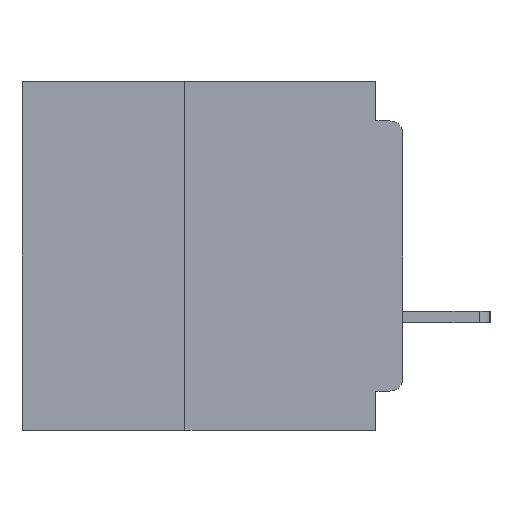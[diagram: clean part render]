
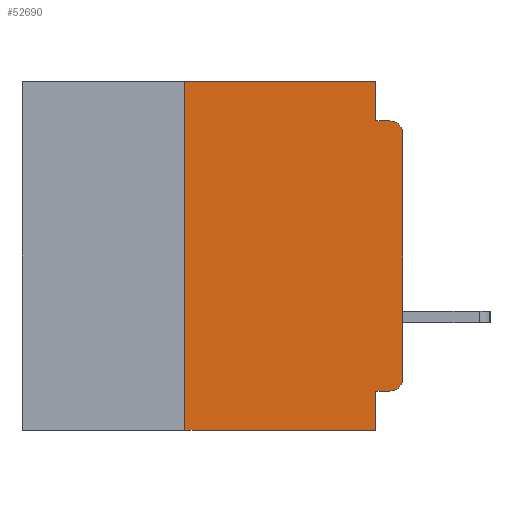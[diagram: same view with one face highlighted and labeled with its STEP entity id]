
A CAD part, left-side view. The second image highlights one B-rep face of the part: STEP entity #52690.
In plain terms, the highlighted planar face has unit normal (-1, 0, 0).
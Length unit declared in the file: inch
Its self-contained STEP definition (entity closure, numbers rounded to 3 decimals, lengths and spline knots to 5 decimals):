
#367 = EDGE_CURVE ( 'NONE', #16451, #44723, #26080, .T. ) ;
#374 = ORIENTED_EDGE ( 'NONE', *, *, #367, .F. ) ;
#392 = CARTESIAN_POINT ( 'NONE',  ( 0., 0., -0.045 ) ) ;
#437 = DIRECTION ( 'NONE',  ( 0., -1., 0. ) ) ;
#832 = VECTOR ( 'NONE', #9213, 39.37008 ) ;
#1749 = VERTEX_POINT ( 'NONE', #26171 ) ;
#2011 = CARTESIAN_POINT ( 'NONE',  ( 0., 0.015, -0.34 ) ) ;
#2758 = EDGE_CURVE ( 'NONE', #1749, #16451, #26442, .T. ) ;
#3378 = ORIENTED_EDGE ( 'NONE', *, *, #36757, .F. ) ;
#4175 = VECTOR ( 'NONE', #52086, 39.37008 ) ;
#4732 = VERTEX_POINT ( 'NONE', #40235 ) ;
#6207 = DIRECTION ( 'NONE',  ( 0., 0., -1. ) ) ;
#6272 = CARTESIAN_POINT ( 'NONE',  ( 0., 0.015, -0.045 ) ) ;
#7562 = CARTESIAN_POINT ( 'NONE',  ( 0., 0.015, -0.355 ) ) ;
#7937 = EDGE_CURVE ( 'NONE', #4732, #1749, #18870, .T. ) ;
#8216 = AXIS2_PLACEMENT_3D ( 'NONE', #2011, #30762, #6207 ) ;
#9036 = FACE_OUTER_BOUND ( 'NONE', #14823, .T. ) ;
#9213 = DIRECTION ( 'NONE',  ( 0., 0., 1. ) ) ;
#10771 = ORIENTED_EDGE ( 'NONE', *, *, #25260, .T. ) ;
#10917 = VERTEX_POINT ( 'NONE', #40753 ) ;
#11067 = CARTESIAN_POINT ( 'NONE',  ( 0., 0.031, -0.045 ) ) ;
#12287 = ORIENTED_EDGE ( 'NONE', *, *, #12559, .T. ) ;
#12559 = EDGE_CURVE ( 'NONE', #31910, #25342, #45530, .T. ) ;
#12578 = DIRECTION ( 'NONE',  ( 0., 0., -1. ) ) ;
#13966 = DIRECTION ( 'NONE',  ( -1., 0., 0. ) ) ;
#14116 = AXIS2_PLACEMENT_3D ( 'NONE', #38330, #13966, #42413 ) ;
#14642 = DIRECTION ( 'NONE',  ( 0., 0., -1. ) ) ;
#14823 = EDGE_LOOP ( 'NONE', ( #10771, #35014, #374, #29290, #21472, #31217, #22870, #3378, #26031, #12287 ) ) ;
#15017 = VERTEX_POINT ( 'NONE', #21821 ) ;
#16313 = LINE ( 'NONE', #24455, #25896 ) ;
#16451 = VERTEX_POINT ( 'NONE', #11067 ) ;
#16553 = CARTESIAN_POINT ( 'NONE',  ( 0., 0.25, -0.4 ) ) ;
#17616 = VECTOR ( 'NONE', #437, 39.37008 ) ;
#18870 = LINE ( 'NONE', #21215, #17616 ) ;
#21215 = CARTESIAN_POINT ( 'NONE',  ( 0., 0.437, 0. ) ) ;
#21472 = ORIENTED_EDGE ( 'NONE', *, *, #7937, .F. ) ;
#21821 = CARTESIAN_POINT ( 'NONE',  ( 0., 0.25, -0.4 ) ) ;
#22835 = VERTEX_POINT ( 'NONE', #41544 ) ;
#22870 = ORIENTED_EDGE ( 'NONE', *, *, #39452, .T. ) ;
#23861 = DIRECTION ( 'NONE',  ( 0., -1., 0. ) ) ;
#24090 = LINE ( 'NONE', #25539, #832 ) ;
#24455 = CARTESIAN_POINT ( 'NONE',  ( 0., 0., -0.355 ) ) ;
#25260 = EDGE_CURVE ( 'NONE', #25342, #10917, #24090, .T. ) ;
#25342 = VERTEX_POINT ( 'NONE', #30139 ) ;
#25539 = CARTESIAN_POINT ( 'NONE',  ( 0., 0., 0. ) ) ;
#25896 = VECTOR ( 'NONE', #28549, 39.37008 ) ;
#26031 = ORIENTED_EDGE ( 'NONE', *, *, #37140, .F. ) ;
#26080 = LINE ( 'NONE', #392, #4175 ) ;
#26171 = CARTESIAN_POINT ( 'NONE',  ( 0., 0.031, 0. ) ) ;
#26278 = EDGE_CURVE ( 'NONE', #10917, #44723, #35391, .T. ) ;
#26442 = LINE ( 'NONE', #51090, #35946 ) ;
#26671 = VECTOR ( 'NONE', #37972, 39.37008 ) ;
#27740 = AXIS2_PLACEMENT_3D ( 'NONE', #32923, #49086, #12578 ) ;
#27935 = LINE ( 'NONE', #50233, #26671 ) ;
#28243 = VECTOR ( 'NONE', #23861, 39.37008 ) ;
#28549 = DIRECTION ( 'NONE',  ( 0., 1., 0. ) ) ;
#29290 = ORIENTED_EDGE ( 'NONE', *, *, #2758, .F. ) ;
#30139 = CARTESIAN_POINT ( 'NONE',  ( 0., 0., -0.34 ) ) ;
#30450 = VECTOR ( 'NONE', #44992, 39.37008 ) ;
#30762 = DIRECTION ( 'NONE',  ( -1., 0., 0. ) ) ;
#31217 = ORIENTED_EDGE ( 'NONE', *, *, #50369, .F. ) ;
#31910 = VERTEX_POINT ( 'NONE', #7562 ) ;
#32923 = CARTESIAN_POINT ( 'NONE',  ( 0., 0.437, 0. ) ) ;
#35014 = ORIENTED_EDGE ( 'NONE', *, *, #26278, .T. ) ;
#35277 = VERTEX_POINT ( 'NONE', #40838 ) ;
#35391 = CIRCLE ( 'NONE', #14116, 0.015 ) ;
#35946 = VECTOR ( 'NONE', #14642, 39.37008 ) ;
#36757 = EDGE_CURVE ( 'NONE', #35277, #22835, #27935, .T. ) ;
#36985 = PLANE ( 'NONE',  #27740 ) ;
#37140 = EDGE_CURVE ( 'NONE', #31910, #35277, #16313, .T. ) ;
#37972 = DIRECTION ( 'NONE',  ( 0., 0., -1. ) ) ;
#38330 = CARTESIAN_POINT ( 'NONE',  ( 0., 0.015, -0.06 ) ) ;
#38999 = LINE ( 'NONE', #40006, #28243 ) ;
#39452 = EDGE_CURVE ( 'NONE', #15017, #22835, #38999, .T. ) ;
#40006 = CARTESIAN_POINT ( 'NONE',  ( 0., 0.437, -0.4 ) ) ;
#40235 = CARTESIAN_POINT ( 'NONE',  ( 0., 0.25, 0. ) ) ;
#40753 = CARTESIAN_POINT ( 'NONE',  ( 0., 0., -0.06 ) ) ;
#40838 = CARTESIAN_POINT ( 'NONE',  ( 0., 0.031, -0.355 ) ) ;
#41234 = LINE ( 'NONE', #16553, #30450 ) ;
#41544 = CARTESIAN_POINT ( 'NONE',  ( 0., 0.031, -0.4 ) ) ;
#42413 = DIRECTION ( 'NONE',  ( 0., 0., -1. ) ) ;
#44723 = VERTEX_POINT ( 'NONE', #6272 ) ;
#44992 = DIRECTION ( 'NONE',  ( 0., 0., 1. ) ) ;
#45530 = CIRCLE ( 'NONE', #8216, 0.015 ) ;
#49086 = DIRECTION ( 'NONE',  ( 1., 0., 0. ) ) ;
#50233 = CARTESIAN_POINT ( 'NONE',  ( 0., 0.031, -0.4 ) ) ;
#50369 = EDGE_CURVE ( 'NONE', #15017, #4732, #41234, .T. ) ;
#51090 = CARTESIAN_POINT ( 'NONE',  ( 0., 0.031, 0. ) ) ;
#52086 = DIRECTION ( 'NONE',  ( 0., -1., 0. ) ) ;
#52690 = ADVANCED_FACE ( 'NONE', ( #9036 ), #36985, .F. ) ;
